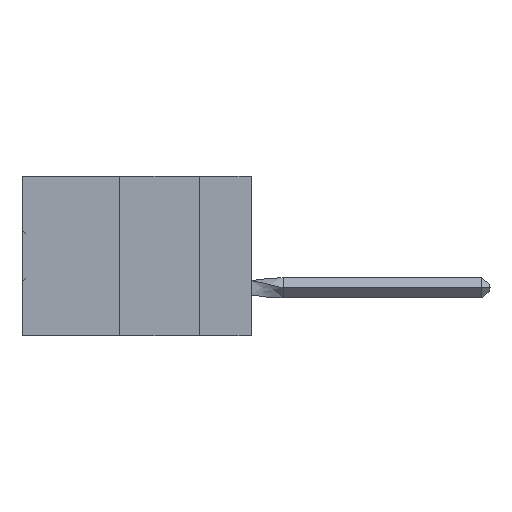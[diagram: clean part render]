
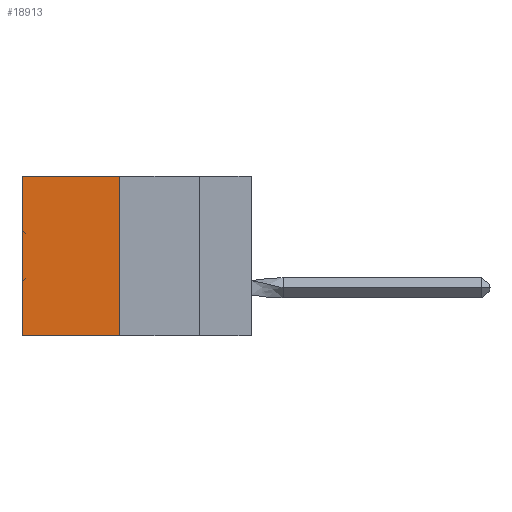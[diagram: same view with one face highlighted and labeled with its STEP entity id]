
A CAD part, left-side view. The second image highlights one B-rep face of the part: STEP entity #18913.
In plain terms, the highlighted planar face has unit normal (-1, 0, 0).
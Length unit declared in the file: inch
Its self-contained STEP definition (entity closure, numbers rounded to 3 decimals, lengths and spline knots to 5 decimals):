
#191 = VERTEX_POINT ( 'NONE', #18562 ) ;
#5000 = CARTESIAN_POINT ( 'NONE',  ( 0.305, 0.72, -0.5 ) ) ;
#5031 = EDGE_CURVE ( 'NONE', #191, #29252, #30286, .T. ) ;
#5594 = DIRECTION ( 'NONE',  ( 0., 0., -1. ) ) ;
#8662 = ORIENTED_EDGE ( 'NONE', *, *, #15449, .T. ) ;
#10997 = DIRECTION ( 'NONE',  ( 1., 0., 0. ) ) ;
#11990 = VERTEX_POINT ( 'NONE', #41598 ) ;
#12017 = CARTESIAN_POINT ( 'NONE',  ( 0.305, 0.413, 0. ) ) ;
#13606 = VECTOR ( 'NONE', #55522, 39.37008 ) ;
#13716 = ORIENTED_EDGE ( 'NONE', *, *, #5031, .F. ) ;
#14272 = EDGE_CURVE ( 'NONE', #191, #27554, #19153, .T. ) ;
#15449 = EDGE_CURVE ( 'NONE', #27554, #11990, #16493, .T. ) ;
#15652 = ORIENTED_EDGE ( 'NONE', *, *, #42392, .F. ) ;
#16493 = LINE ( 'NONE', #5000, #13606 ) ;
#16723 = FACE_OUTER_BOUND ( 'NONE', #27236, .T. ) ;
#17261 = CARTESIAN_POINT ( 'NONE',  ( 0.305, 0.413, -0.5 ) ) ;
#18562 = CARTESIAN_POINT ( 'NONE',  ( 0.305, 0.413, 0. ) ) ;
#18913 = ADVANCED_FACE ( 'NONE', ( #16723 ), #33687, .F. ) ;
#19153 = LINE ( 'NONE', #12017, #28462 ) ;
#22061 = DIRECTION ( 'NONE',  ( 0., 1., 0. ) ) ;
#23212 = AXIS2_PLACEMENT_3D ( 'NONE', #33096, #10997, #5594 ) ;
#27236 = EDGE_LOOP ( 'NONE', ( #8662, #15652, #13716, #57288 ) ) ;
#27554 = VERTEX_POINT ( 'NONE', #52064 ) ;
#28462 = VECTOR ( 'NONE', #40065, 39.37008 ) ;
#28625 = DIRECTION ( 'NONE',  ( 0., 0., -1. ) ) ;
#28864 = VECTOR ( 'NONE', #28625, 39.37008 ) ;
#29252 = VERTEX_POINT ( 'NONE', #43753 ) ;
#30286 = LINE ( 'NONE', #55447, #28864 ) ;
#33096 = CARTESIAN_POINT ( 'NONE',  ( 0.305, 0.413, -0.5 ) ) ;
#33687 = PLANE ( 'NONE',  #23212 ) ;
#37211 = VECTOR ( 'NONE', #22061, 39.37008 ) ;
#40065 = DIRECTION ( 'NONE',  ( 0., 1., 0. ) ) ;
#41598 = CARTESIAN_POINT ( 'NONE',  ( 0.305, 0.72, -0.5 ) ) ;
#42392 = EDGE_CURVE ( 'NONE', #29252, #11990, #49360, .T. ) ;
#43753 = CARTESIAN_POINT ( 'NONE',  ( 0.305, 0.413, -0.5 ) ) ;
#49360 = LINE ( 'NONE', #17261, #37211 ) ;
#52064 = CARTESIAN_POINT ( 'NONE',  ( 0.305, 0.72, 0. ) ) ;
#55447 = CARTESIAN_POINT ( 'NONE',  ( 0.305, 0.413, -0.5 ) ) ;
#55522 = DIRECTION ( 'NONE',  ( 0., 0., -1. ) ) ;
#57288 = ORIENTED_EDGE ( 'NONE', *, *, #14272, .T. ) ;
